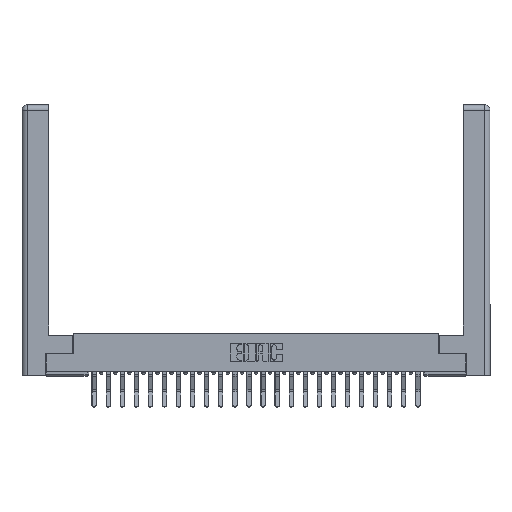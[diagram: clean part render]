
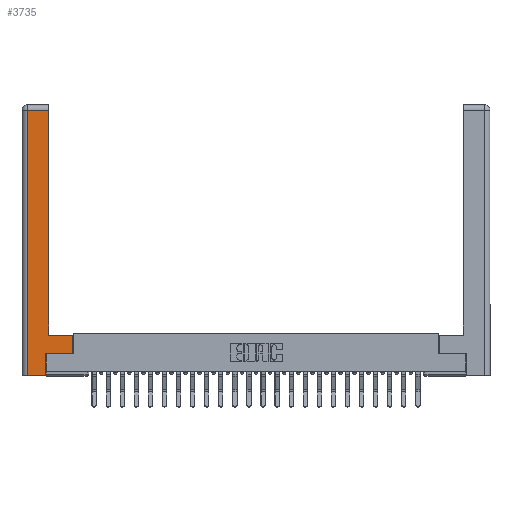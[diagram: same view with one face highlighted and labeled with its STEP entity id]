
A CAD part, top view. The second image highlights one B-rep face of the part: STEP entity #3735.
In plain terms, the highlighted planar face has unit normal (0, 0, 1).
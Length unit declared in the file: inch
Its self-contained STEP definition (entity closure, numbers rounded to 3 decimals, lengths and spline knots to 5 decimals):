
#60 = ORIENTED_EDGE ( 'NONE', *, *, #12182, .T. ) ;
#625 = DIRECTION ( 'NONE',  ( -1., 0., 0. ) ) ;
#895 = CARTESIAN_POINT ( 'NONE',  ( 0.0615, 2.94, 0. ) ) ;
#1489 = ORIENTED_EDGE ( 'NONE', *, *, #10345, .T. ) ;
#2151 = ORIENTED_EDGE ( 'NONE', *, *, #8662, .T. ) ;
#2368 = CARTESIAN_POINT ( 'NONE',  ( 0.265, 0., 0. ) ) ;
#2917 = CARTESIAN_POINT ( 'NONE',  ( 0.565, 0.245, 0. ) ) ;
#2939 = ORIENTED_EDGE ( 'NONE', *, *, #13531, .T. ) ;
#3147 = DIRECTION ( 'NONE',  ( 1., 0., 0. ) ) ;
#3371 = CARTESIAN_POINT ( 'NONE',  ( 0.0615, 0., 0. ) ) ;
#3735 = ADVANCED_FACE ( 'NONE', ( #20696 ), #6308, .F. ) ;
#4653 = LINE ( 'NONE', #12773, #16941 ) ;
#5132 = LINE ( 'NONE', #23502, #5837 ) ;
#5142 = VECTOR ( 'NONE', #24606, 39.37008 ) ;
#5266 = DIRECTION ( 'NONE',  ( -1., 0., 0. ) ) ;
#5647 = VERTEX_POINT ( 'NONE', #14269 ) ;
#5837 = VECTOR ( 'NONE', #5266, 39.37008 ) ;
#6299 = VERTEX_POINT ( 'NONE', #15883 ) ;
#6308 = PLANE ( 'NONE',  #25033 ) ;
#6662 = ORIENTED_EDGE ( 'NONE', *, *, #21908, .T. ) ;
#7901 = DIRECTION ( 'NONE',  ( 0., -1., 0. ) ) ;
#8662 = EDGE_CURVE ( 'NONE', #20307, #21671, #15793, .T. ) ;
#8839 = EDGE_LOOP ( 'NONE', ( #16602, #60, #16339, #6662, #1489, #2151, #2939, #22579 ) ) ;
#9047 = DIRECTION ( 'NONE',  ( 0., 1., 0. ) ) ;
#10345 = EDGE_CURVE ( 'NONE', #6299, #20307, #16780, .T. ) ;
#10409 = VERTEX_POINT ( 'NONE', #16905 ) ;
#10775 = CARTESIAN_POINT ( 'NONE',  ( 0.0615, 2.94, 0. ) ) ;
#10859 = EDGE_CURVE ( 'NONE', #5647, #13996, #5132, .T. ) ;
#12182 = EDGE_CURVE ( 'NONE', #22374, #15864, #16754, .T. ) ;
#12550 = CARTESIAN_POINT ( 'NONE',  ( 0.265, 0.245, 0. ) ) ;
#12773 = CARTESIAN_POINT ( 'NONE',  ( 0.565, 0.45, 0. ) ) ;
#12877 = CARTESIAN_POINT ( 'NONE',  ( 0.265, 0.245, 0. ) ) ;
#13034 = CARTESIAN_POINT ( 'NONE',  ( 0.295, 3., 0. ) ) ;
#13531 = EDGE_CURVE ( 'NONE', #21671, #5647, #4653, .T. ) ;
#13996 = VERTEX_POINT ( 'NONE', #18605 ) ;
#14269 = CARTESIAN_POINT ( 'NONE',  ( 0.565, 0.45, 0. ) ) ;
#15065 = VECTOR ( 'NONE', #3147, 39.37008 ) ;
#15128 = EDGE_CURVE ( 'NONE', #15864, #10409, #26135, .T. ) ;
#15393 = CARTESIAN_POINT ( 'NONE',  ( 0.295, 2.94, 0. ) ) ;
#15793 = LINE ( 'NONE', #17392, #15065 ) ;
#15864 = VERTEX_POINT ( 'NONE', #895 ) ;
#15883 = CARTESIAN_POINT ( 'NONE',  ( 0.265, 0., 0. ) ) ;
#15954 = LINE ( 'NONE', #2368, #5142 ) ;
#16339 = ORIENTED_EDGE ( 'NONE', *, *, #15128, .T. ) ;
#16602 = ORIENTED_EDGE ( 'NONE', *, *, #21670, .T. ) ;
#16754 = LINE ( 'NONE', #10775, #25887 ) ;
#16780 = LINE ( 'NONE', #12550, #21547 ) ;
#16892 = LINE ( 'NONE', #13034, #19574 ) ;
#16905 = CARTESIAN_POINT ( 'NONE',  ( 0.0615, 0., 0. ) ) ;
#16941 = VECTOR ( 'NONE', #9047, 39.37008 ) ;
#17392 = CARTESIAN_POINT ( 'NONE',  ( 0.565, 0.245, 0. ) ) ;
#18605 = CARTESIAN_POINT ( 'NONE',  ( 0.295, 0.45, 0. ) ) ;
#18822 = CARTESIAN_POINT ( 'NONE',  ( 0., 0., 0. ) ) ;
#19574 = VECTOR ( 'NONE', #21156, 39.37008 ) ;
#20307 = VERTEX_POINT ( 'NONE', #12877 ) ;
#20438 = DIRECTION ( 'NONE',  ( 0., 0., -1. ) ) ;
#20696 = FACE_OUTER_BOUND ( 'NONE', #8839, .T. ) ;
#20795 = DIRECTION ( 'NONE',  ( 0., 1., 0. ) ) ;
#21027 = VECTOR ( 'NONE', #7901, 39.37008 ) ;
#21156 = DIRECTION ( 'NONE',  ( 0., 1., 0. ) ) ;
#21547 = VECTOR ( 'NONE', #20795, 39.37008 ) ;
#21670 = EDGE_CURVE ( 'NONE', #13996, #22374, #16892, .T. ) ;
#21671 = VERTEX_POINT ( 'NONE', #2917 ) ;
#21908 = EDGE_CURVE ( 'NONE', #10409, #6299, #15954, .T. ) ;
#22374 = VERTEX_POINT ( 'NONE', #15393 ) ;
#22552 = DIRECTION ( 'NONE',  ( -1., 0., 0. ) ) ;
#22579 = ORIENTED_EDGE ( 'NONE', *, *, #10859, .T. ) ;
#23502 = CARTESIAN_POINT ( 'NONE',  ( 0.295, 0.45, 0. ) ) ;
#24606 = DIRECTION ( 'NONE',  ( 1., 0., 0. ) ) ;
#25033 = AXIS2_PLACEMENT_3D ( 'NONE', #18822, #20438, #22552 ) ;
#25887 = VECTOR ( 'NONE', #625, 39.37008 ) ;
#26135 = LINE ( 'NONE', #3371, #21027 ) ;
